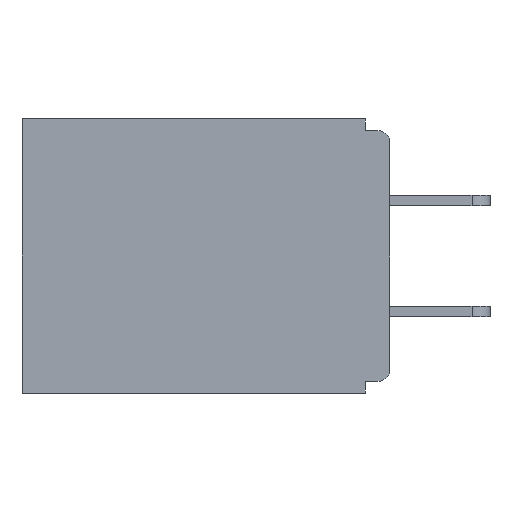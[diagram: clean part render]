
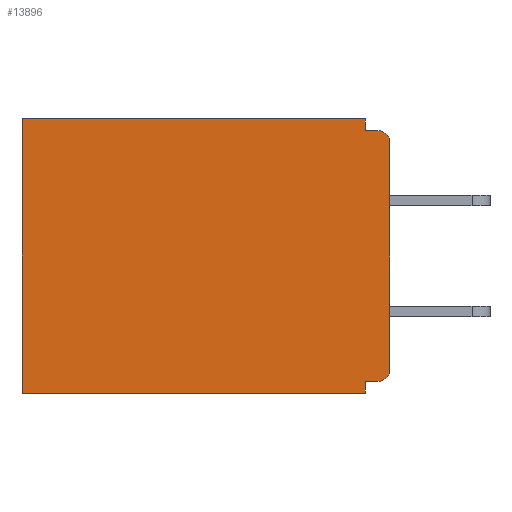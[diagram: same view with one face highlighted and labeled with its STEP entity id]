
A CAD part, left-side view. The second image highlights one B-rep face of the part: STEP entity #13896.
In plain terms, the highlighted planar face has unit normal (-1, 0, 0).
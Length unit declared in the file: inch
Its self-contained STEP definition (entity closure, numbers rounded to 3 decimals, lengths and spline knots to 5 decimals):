
#564 = VERTEX_POINT ( 'NONE', #5057 ) ;
#736 = CARTESIAN_POINT ( 'NONE',  ( 0.298, 0.031, -0.015 ) ) ;
#777 = VECTOR ( 'NONE', #22357, 39.37008 ) ;
#855 = DIRECTION ( 'NONE',  ( 0., 1., 0. ) ) ;
#1025 = EDGE_CURVE ( 'NONE', #564, #6738, #5268, .T. ) ;
#1490 = DIRECTION ( 'NONE',  ( 0., 0., -1. ) ) ;
#1563 = CARTESIAN_POINT ( 'NONE',  ( 0.298, 0., -0.343 ) ) ;
#1650 = LINE ( 'NONE', #27329, #23159 ) ;
#1789 = VERTEX_POINT ( 'NONE', #736 ) ;
#1995 = EDGE_CURVE ( 'NONE', #12804, #28348, #23119, .T. ) ;
#2054 = DIRECTION ( 'NONE',  ( 0., 0., -1. ) ) ;
#3503 = VECTOR ( 'NONE', #10190, 39.37008 ) ;
#3862 = ORIENTED_EDGE ( 'NONE', *, *, #13474, .F. ) ;
#5057 = CARTESIAN_POINT ( 'NONE',  ( 0.298, 0.015, -0.328 ) ) ;
#5268 = LINE ( 'NONE', #17066, #16709 ) ;
#5704 = CARTESIAN_POINT ( 'NONE',  ( 0.298, 0., -0.015 ) ) ;
#5746 = EDGE_LOOP ( 'NONE', ( #23251, #9586, #3862, #11172, #13471, #21851, #17823, #16755, #12418, #6519 ) ) ;
#5883 = VERTEX_POINT ( 'NONE', #17826 ) ;
#6090 = LINE ( 'NONE', #5704, #24493 ) ;
#6115 = VECTOR ( 'NONE', #855, 39.37008 ) ;
#6139 = LINE ( 'NONE', #18554, #26628 ) ;
#6444 = CARTESIAN_POINT ( 'NONE',  ( 0.298, 0., 0. ) ) ;
#6519 = ORIENTED_EDGE ( 'NONE', *, *, #26770, .F. ) ;
#6612 = EDGE_CURVE ( 'NONE', #8466, #9126, #26939, .T. ) ;
#6738 = VERTEX_POINT ( 'NONE', #21466 ) ;
#6784 = LINE ( 'NONE', #9695, #6115 ) ;
#6811 = DIRECTION ( 'NONE',  ( 0., 0., -1. ) ) ;
#6892 = AXIS2_PLACEMENT_3D ( 'NONE', #6444, #20152, #6811 ) ;
#7444 = CARTESIAN_POINT ( 'NONE',  ( 0.298, 0., -0.03 ) ) ;
#7565 = CARTESIAN_POINT ( 'NONE',  ( 0.298, 0.46, -0.343 ) ) ;
#7798 = VERTEX_POINT ( 'NONE', #9630 ) ;
#8466 = VERTEX_POINT ( 'NONE', #7444 ) ;
#9126 = VERTEX_POINT ( 'NONE', #26335 ) ;
#9142 = EDGE_CURVE ( 'NONE', #6738, #7798, #14753, .T. ) ;
#9586 = ORIENTED_EDGE ( 'NONE', *, *, #23823, .F. ) ;
#9630 = CARTESIAN_POINT ( 'NONE',  ( 0.298, 0.031, -0.343 ) ) ;
#9695 = CARTESIAN_POINT ( 'NONE',  ( 0.298, 0., 0. ) ) ;
#10070 = DIRECTION ( 'NONE',  ( 0., 0., -1. ) ) ;
#10190 = DIRECTION ( 'NONE',  ( 0., 1., 0. ) ) ;
#10687 = DIRECTION ( 'NONE',  ( 0., 0., -1. ) ) ;
#10851 = EDGE_CURVE ( 'NONE', #564, #5883, #22602, .T. ) ;
#11172 = ORIENTED_EDGE ( 'NONE', *, *, #23439, .T. ) ;
#11192 = EDGE_CURVE ( 'NONE', #7798, #28348, #27407, .T. ) ;
#12418 = ORIENTED_EDGE ( 'NONE', *, *, #10851, .T. ) ;
#12804 = VERTEX_POINT ( 'NONE', #14600 ) ;
#13289 = VERTEX_POINT ( 'NONE', #22662 ) ;
#13471 = ORIENTED_EDGE ( 'NONE', *, *, #1995, .T. ) ;
#13474 = EDGE_CURVE ( 'NONE', #13289, #1789, #1650, .T. ) ;
#13896 = ADVANCED_FACE ( 'NONE', ( #16683 ), #22180, .F. ) ;
#14600 = CARTESIAN_POINT ( 'NONE',  ( 0.298, 0.46, 0. ) ) ;
#14753 = LINE ( 'NONE', #24663, #777 ) ;
#16136 = AXIS2_PLACEMENT_3D ( 'NONE', #27885, #16680, #10070 ) ;
#16680 = DIRECTION ( 'NONE',  ( -1., 0., 0. ) ) ;
#16683 = FACE_OUTER_BOUND ( 'NONE', #5746, .T. ) ;
#16709 = VECTOR ( 'NONE', #16775, 39.37008 ) ;
#16755 = ORIENTED_EDGE ( 'NONE', *, *, #1025, .F. ) ;
#16775 = DIRECTION ( 'NONE',  ( 0., 1., 0. ) ) ;
#16799 = CARTESIAN_POINT ( 'NONE',  ( 0.298, 0.46, 0. ) ) ;
#17066 = CARTESIAN_POINT ( 'NONE',  ( 0.298, 0., -0.328 ) ) ;
#17652 = AXIS2_PLACEMENT_3D ( 'NONE', #21003, #18966, #1490 ) ;
#17823 = ORIENTED_EDGE ( 'NONE', *, *, #9142, .F. ) ;
#17826 = CARTESIAN_POINT ( 'NONE',  ( 0.298, 0., -0.313 ) ) ;
#18309 = DIRECTION ( 'NONE',  ( 0., 0., -1. ) ) ;
#18554 = CARTESIAN_POINT ( 'NONE',  ( 0.298, 0., 0. ) ) ;
#18966 = DIRECTION ( 'NONE',  ( -1., 0., 0. ) ) ;
#20152 = DIRECTION ( 'NONE',  ( 1., 0., 0. ) ) ;
#21003 = CARTESIAN_POINT ( 'NONE',  ( 0.298, 0.015, -0.03 ) ) ;
#21466 = CARTESIAN_POINT ( 'NONE',  ( 0.298, 0.031, -0.328 ) ) ;
#21851 = ORIENTED_EDGE ( 'NONE', *, *, #11192, .F. ) ;
#22180 = PLANE ( 'NONE',  #6892 ) ;
#22357 = DIRECTION ( 'NONE',  ( 0., 0., -1. ) ) ;
#22602 = CIRCLE ( 'NONE', #16136, 0.015 ) ;
#22662 = CARTESIAN_POINT ( 'NONE',  ( 0.298, 0.031, 0. ) ) ;
#23119 = LINE ( 'NONE', #16799, #28275 ) ;
#23159 = VECTOR ( 'NONE', #18309, 39.37008 ) ;
#23251 = ORIENTED_EDGE ( 'NONE', *, *, #6612, .T. ) ;
#23439 = EDGE_CURVE ( 'NONE', #13289, #12804, #6784, .T. ) ;
#23823 = EDGE_CURVE ( 'NONE', #1789, #9126, #6090, .T. ) ;
#24493 = VECTOR ( 'NONE', #25308, 39.37008 ) ;
#24663 = CARTESIAN_POINT ( 'NONE',  ( 0.298, 0.031, -0.343 ) ) ;
#25308 = DIRECTION ( 'NONE',  ( 0., -1., 0. ) ) ;
#26335 = CARTESIAN_POINT ( 'NONE',  ( 0.298, 0.015, -0.015 ) ) ;
#26628 = VECTOR ( 'NONE', #2054, 39.37008 ) ;
#26770 = EDGE_CURVE ( 'NONE', #8466, #5883, #6139, .T. ) ;
#26939 = CIRCLE ( 'NONE', #17652, 0.015 ) ;
#27329 = CARTESIAN_POINT ( 'NONE',  ( 0.298, 0.031, -0.343 ) ) ;
#27407 = LINE ( 'NONE', #1563, #3503 ) ;
#27885 = CARTESIAN_POINT ( 'NONE',  ( 0.298, 0.015, -0.313 ) ) ;
#28275 = VECTOR ( 'NONE', #10687, 39.37008 ) ;
#28348 = VERTEX_POINT ( 'NONE', #7565 ) ;
